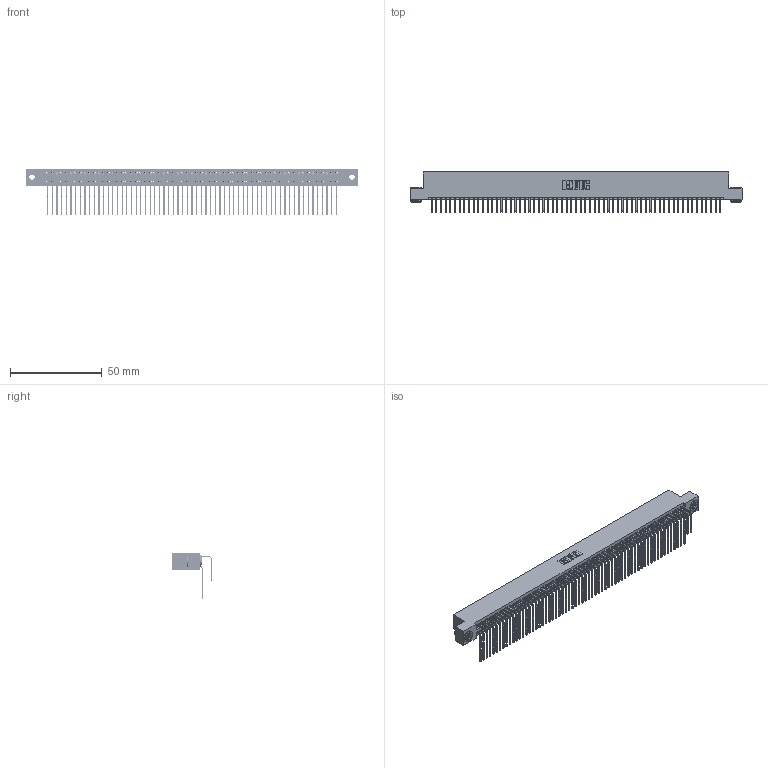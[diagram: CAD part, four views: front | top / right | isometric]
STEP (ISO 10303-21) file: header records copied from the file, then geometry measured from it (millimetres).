
FILE_DESCRIPTION (( 'STEP AP203' ), '1' );
FILE_NAME ('395-126-558-203.STEP', '2019-10-28T16:36:58', ( '' ), ( '' ), 'SwSTEP 2.0', 'SolidWorks 2016', '' );
FILE_SCHEMA (( 'CONFIG_CONTROL_DESIGN' ));
Length unit declared in the file: inch
Products named in the file (5): 395-126-558-203; 345 Part_Flush Mounting Lugs - 0.156 Dia-TH; 345-292-001_558 559 Tail - 1; 345-292-001_558 Tail - 2; 345-250-002_345-250-002-102
Assembly tree (129 placements, depth 2):
  395-126-558-203
    345 Part_Flush Mounting Lugs - 0.156 Dia-TH
    345-292-001_558 559 Tail - 1  x63
    345-292-001_558 Tail - 2  x63
    345-250-002_345-250-002-102  x2
Bounding box: 181.23 x 21.83 x 25.53 mm (x, y, z)
Volume: 18546 mm3; surface area: 31443.6 mm2
Topology: 129 solids, 129 shells, 6716 faces, 19947 edges, 13126 vertices
Faces by surface type: plane 4500, cylinder 2208, cone 8
Entity records: 48906 total; most frequent: CARTESIAN_POINT 8198, ORIENTED_EDGE 8074, DIRECTION 7207, EDGE_CURVE 4037, LINE 3589, VECTOR 3589, VERTEX_POINT 2686, AXIS2_PLACEMENT_3D 1809
